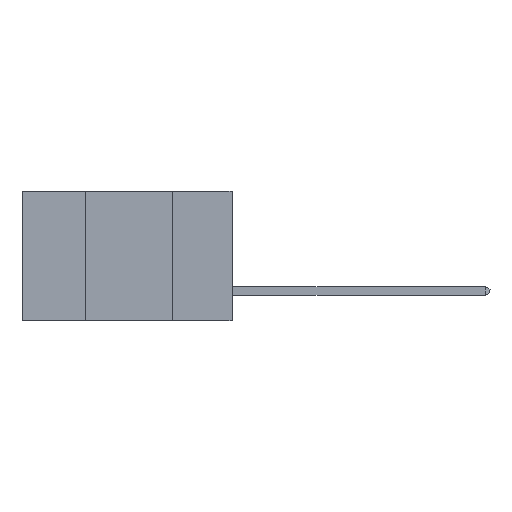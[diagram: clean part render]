
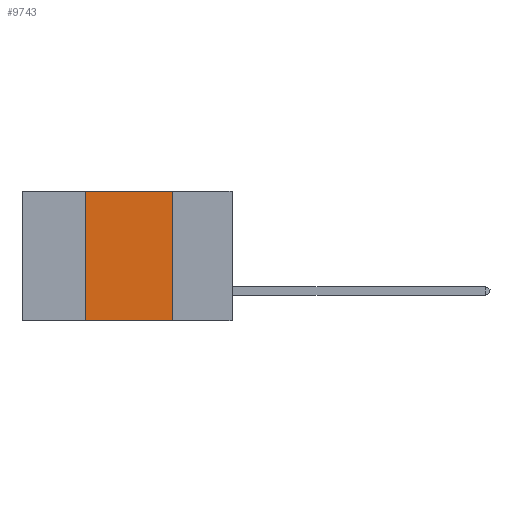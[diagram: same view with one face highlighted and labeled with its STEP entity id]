
A CAD part, left-side view. The second image highlights one B-rep face of the part: STEP entity #9743.
In plain terms, the highlighted planar face has unit normal (-1, 0, 0).
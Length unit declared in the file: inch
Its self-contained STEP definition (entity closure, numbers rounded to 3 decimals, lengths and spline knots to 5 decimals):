
#35 = EDGE_CURVE ( 'NONE', #9546, #4440, #6831, .T. ) ;
#101 = ORIENTED_EDGE ( 'NONE', *, *, #5337, .T. ) ;
#613 = CARTESIAN_POINT ( 'NONE',  ( 0., 0.42, -0.37 ) ) ;
#1233 = CARTESIAN_POINT ( 'NONE',  ( 0., 0.42, 0. ) ) ;
#1377 = EDGE_CURVE ( 'NONE', #4440, #2042, #6626, .T. ) ;
#1587 = VERTEX_POINT ( 'NONE', #11075 ) ;
#1891 = VECTOR ( 'NONE', #2109, 39.37008 ) ;
#1971 = ORIENTED_EDGE ( 'NONE', *, *, #35, .F. ) ;
#2042 = VERTEX_POINT ( 'NONE', #3043 ) ;
#2109 = DIRECTION ( 'NONE',  ( 0., 0., -1. ) ) ;
#3043 = CARTESIAN_POINT ( 'NONE',  ( 0., 0.17, 0. ) ) ;
#4440 = VERTEX_POINT ( 'NONE', #12406 ) ;
#4757 = LINE ( 'NONE', #11437, #1891 ) ;
#5337 = EDGE_CURVE ( 'NONE', #9546, #1587, #9508, .T. ) ;
#5499 = DIRECTION ( 'NONE',  ( 0., 0., -1. ) ) ;
#6383 = ORIENTED_EDGE ( 'NONE', *, *, #1377, .F. ) ;
#6453 = CARTESIAN_POINT ( 'NONE',  ( 0., 0.6, 0. ) ) ;
#6626 = LINE ( 'NONE', #10331, #8062 ) ;
#6831 = LINE ( 'NONE', #1233, #8898 ) ;
#7395 = EDGE_LOOP ( 'NONE', ( #11523, #6383, #1971, #101 ) ) ;
#7882 = DIRECTION ( 'NONE',  ( 0., -1., 0. ) ) ;
#8062 = VECTOR ( 'NONE', #9378, 39.37008 ) ;
#8436 = DIRECTION ( 'NONE',  ( 0., 0., 1. ) ) ;
#8549 = FACE_OUTER_BOUND ( 'NONE', #7395, .T. ) ;
#8898 = VECTOR ( 'NONE', #8436, 39.37008 ) ;
#9378 = DIRECTION ( 'NONE',  ( 0., -1., 0. ) ) ;
#9508 = LINE ( 'NONE', #12759, #11593 ) ;
#9546 = VERTEX_POINT ( 'NONE', #613 ) ;
#9743 = ADVANCED_FACE ( 'NONE', ( #8549 ), #12541, .F. ) ;
#10331 = CARTESIAN_POINT ( 'NONE',  ( 0., 0.6, 0. ) ) ;
#11075 = CARTESIAN_POINT ( 'NONE',  ( 0., 0.17, -0.37 ) ) ;
#11437 = CARTESIAN_POINT ( 'NONE',  ( 0., 0.17, 0. ) ) ;
#11523 = ORIENTED_EDGE ( 'NONE', *, *, #12954, .F. ) ;
#11593 = VECTOR ( 'NONE', #7882, 39.37008 ) ;
#11651 = DIRECTION ( 'NONE',  ( 1., 0., 0. ) ) ;
#11907 = AXIS2_PLACEMENT_3D ( 'NONE', #6453, #11651, #5499 ) ;
#12406 = CARTESIAN_POINT ( 'NONE',  ( 0., 0.42, 0. ) ) ;
#12541 = PLANE ( 'NONE',  #11907 ) ;
#12759 = CARTESIAN_POINT ( 'NONE',  ( 0., 0.6, -0.37 ) ) ;
#12954 = EDGE_CURVE ( 'NONE', #2042, #1587, #4757, .T. ) ;
